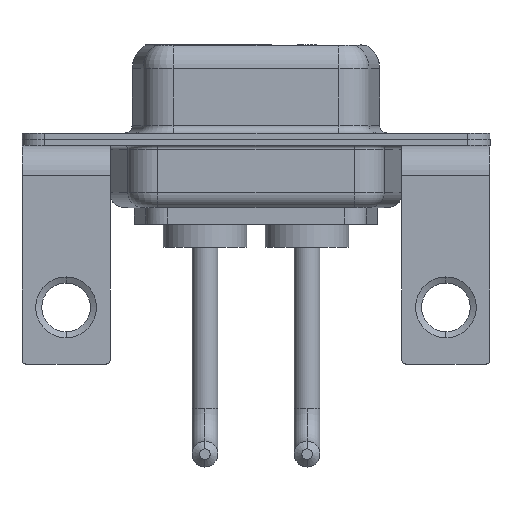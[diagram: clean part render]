
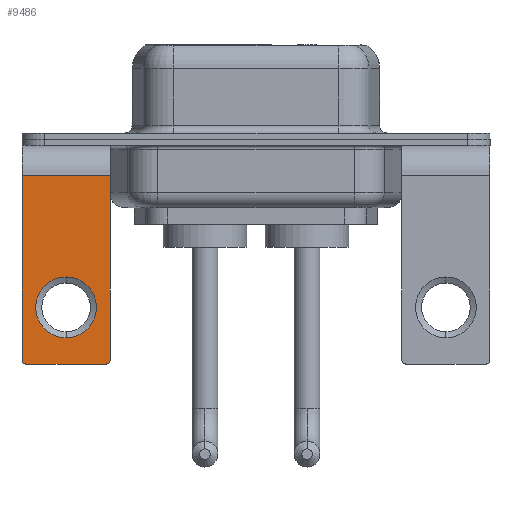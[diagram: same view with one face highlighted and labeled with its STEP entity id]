
A CAD part, front view. The second image highlights one B-rep face of the part: STEP entity #9486.
In plain terms, the highlighted planar face has unit normal (0, -1, 0).
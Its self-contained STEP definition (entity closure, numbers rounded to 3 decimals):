
#219 = EDGE_CURVE ( 'NONE', #10585, #8236, #5377, .T. ) ;
#241 = VERTEX_POINT ( 'NONE', #9851 ) ;
#375 = ORIENTED_EDGE ( 'NONE', *, *, #4380, .T. ) ;
#727 = CARTESIAN_POINT ( 'NONE',  ( 2.9, -6.25, -2.4 ) ) ;
#735 = LINE ( 'NONE', #5100, #12474 ) ;
#761 = EDGE_CURVE ( 'NONE', #241, #4836, #11527, .T. ) ;
#984 = EDGE_LOOP ( 'NONE', ( #2372, #1024, #3324, #11245, #8845, #375 ) ) ;
#1024 = ORIENTED_EDGE ( 'NONE', *, *, #3519, .T. ) ;
#1153 = FACE_BOUND ( 'NONE', #1971, .T. ) ;
#1218 = DIRECTION ( 'NONE',  ( 0., 0., 1. ) ) ;
#1288 = CARTESIAN_POINT ( 'NONE',  ( -2.9, -6.25, -2.4 ) ) ;
#1351 = DIRECTION ( 'NONE',  ( 0., 0., 1. ) ) ;
#1747 = AXIS2_PLACEMENT_3D ( 'NONE', #5234, #8649, #7438 ) ;
#1892 = DIRECTION ( 'NONE',  ( 0., 1., 0. ) ) ;
#1971 = EDGE_LOOP ( 'NONE', ( #13125, #7172 ) ) ;
#1987 = VECTOR ( 'NONE', #5644, 1000. ) ;
#2148 = EDGE_CURVE ( 'NONE', #9730, #10428, #3574, .T. ) ;
#2154 = FACE_OUTER_BOUND ( 'NONE', #984, .T. ) ;
#2372 = ORIENTED_EDGE ( 'NONE', *, *, #2148, .T. ) ;
#2526 = LINE ( 'NONE', #3876, #6105 ) ;
#3103 = EDGE_CURVE ( 'NONE', #4836, #241, #9724, .T. ) ;
#3324 = ORIENTED_EDGE ( 'NONE', *, *, #10625, .F. ) ;
#3519 = EDGE_CURVE ( 'NONE', #10428, #3691, #4720, .T. ) ;
#3564 = AXIS2_PLACEMENT_3D ( 'NONE', #6394, #1892, #8517 ) ;
#3574 = LINE ( 'NONE', #1288, #1987 ) ;
#3691 = VERTEX_POINT ( 'NONE', #5836 ) ;
#3731 = DIRECTION ( 'NONE',  ( -1., 0., 0. ) ) ;
#3869 = CARTESIAN_POINT ( 'NONE',  ( 2.9, -6.25, -14.8 ) ) ;
#3876 = CARTESIAN_POINT ( 'NONE',  ( 2.9, -6.25, -2.4 ) ) ;
#4380 = EDGE_CURVE ( 'NONE', #11723, #9730, #735, .T. ) ;
#4720 = CIRCLE ( 'NONE', #1747, 0.25 ) ;
#4736 = CARTESIAN_POINT ( 'NONE',  ( -2.9, -6.25, -14.55 ) ) ;
#4836 = VERTEX_POINT ( 'NONE', #12264 ) ;
#4858 = CARTESIAN_POINT ( 'NONE',  ( 2.9, -6.25, -14.55 ) ) ;
#4915 = CARTESIAN_POINT ( 'NONE',  ( -2.9, -6.25, -2.4 ) ) ;
#5100 = CARTESIAN_POINT ( 'NONE',  ( 2.9, -6.25, -2.4 ) ) ;
#5234 = CARTESIAN_POINT ( 'NONE',  ( -2.65, -6.25, -14.55 ) ) ;
#5377 = CIRCLE ( 'NONE', #11288, 0.25 ) ;
#5644 = DIRECTION ( 'NONE',  ( 0., 0., -1. ) ) ;
#5836 = CARTESIAN_POINT ( 'NONE',  ( -2.65, -6.25, -14.8 ) ) ;
#5843 = DIRECTION ( 'NONE',  ( 0., 1., 0. ) ) ;
#6105 = VECTOR ( 'NONE', #11517, 1000. ) ;
#6278 = DIRECTION ( 'NONE',  ( 0., 0., 1. ) ) ;
#6394 = CARTESIAN_POINT ( 'NONE',  ( 0., -6.25, -11.07 ) ) ;
#6504 = CARTESIAN_POINT ( 'NONE',  ( 2.9, -6.25, -2.4 ) ) ;
#7172 = ORIENTED_EDGE ( 'NONE', *, *, #761, .T. ) ;
#7420 = DIRECTION ( 'NONE',  ( 0., -1., 0. ) ) ;
#7438 = DIRECTION ( 'NONE',  ( 0., 0., 1. ) ) ;
#7703 = PLANE ( 'NONE',  #11206 ) ;
#8236 = VERTEX_POINT ( 'NONE', #4858 ) ;
#8276 = VECTOR ( 'NONE', #3731, 1000. ) ;
#8517 = DIRECTION ( 'NONE',  ( 0., 0., 1. ) ) ;
#8649 = DIRECTION ( 'NONE',  ( 0., -1., 0. ) ) ;
#8845 = ORIENTED_EDGE ( 'NONE', *, *, #11620, .F. ) ;
#9427 = CARTESIAN_POINT ( 'NONE',  ( 2.65, -6.25, -14.8 ) ) ;
#9445 = DIRECTION ( 'NONE',  ( -1., 0., 0. ) ) ;
#9486 = ADVANCED_FACE ( 'NONE', ( #1153, #2154 ), #7703, .F. ) ;
#9724 = CIRCLE ( 'NONE', #3564, 2. ) ;
#9730 = VERTEX_POINT ( 'NONE', #4915 ) ;
#9851 = CARTESIAN_POINT ( 'NONE',  ( 0., -6.25, -9.07 ) ) ;
#10428 = VERTEX_POINT ( 'NONE', #4736 ) ;
#10585 = VERTEX_POINT ( 'NONE', #9427 ) ;
#10625 = EDGE_CURVE ( 'NONE', #10585, #3691, #13481, .T. ) ;
#10872 = DIRECTION ( 'NONE',  ( 0., 1., 0. ) ) ;
#11206 = AXIS2_PLACEMENT_3D ( 'NONE', #6504, #10872, #1218 ) ;
#11245 = ORIENTED_EDGE ( 'NONE', *, *, #219, .T. ) ;
#11288 = AXIS2_PLACEMENT_3D ( 'NONE', #11927, #7420, #6278 ) ;
#11297 = AXIS2_PLACEMENT_3D ( 'NONE', #13321, #5843, #1351 ) ;
#11517 = DIRECTION ( 'NONE',  ( 0., 0., -1. ) ) ;
#11527 = CIRCLE ( 'NONE', #11297, 2. ) ;
#11620 = EDGE_CURVE ( 'NONE', #11723, #8236, #2526, .T. ) ;
#11723 = VERTEX_POINT ( 'NONE', #727 ) ;
#11927 = CARTESIAN_POINT ( 'NONE',  ( 2.65, -6.25, -14.55 ) ) ;
#12264 = CARTESIAN_POINT ( 'NONE',  ( 0., -6.25, -13.07 ) ) ;
#12474 = VECTOR ( 'NONE', #9445, 1000. ) ;
#13125 = ORIENTED_EDGE ( 'NONE', *, *, #3103, .T. ) ;
#13321 = CARTESIAN_POINT ( 'NONE',  ( 0., -6.25, -11.07 ) ) ;
#13481 = LINE ( 'NONE', #3869, #8276 ) ;
